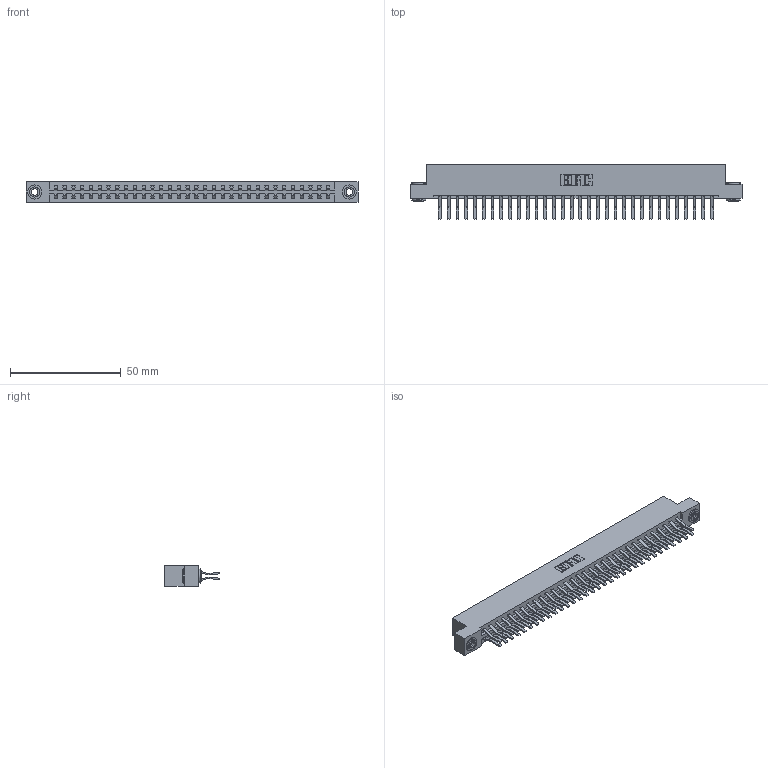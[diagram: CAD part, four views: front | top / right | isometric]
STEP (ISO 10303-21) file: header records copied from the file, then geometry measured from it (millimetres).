
FILE_DESCRIPTION (( 'STEP AP203' ), '1' );
FILE_NAME ('387-064-560-203.STEP', '2019-10-19T17:47:14', ( '' ), ( '' ), 'SwSTEP 2.0', 'SolidWorks 2016', '' );
FILE_SCHEMA (( 'CONFIG_CONTROL_DESIGN' ));
Length unit declared in the file: inch
Products named in the file (4): 345-250-002_345-250-002-102; 387-064-560-203; 337 Part_Flush Mounting Lugs - 0.156 Dia-TH; 345-292-001_560 Tail
Assembly tree (67 placements, depth 2):
  387-064-560-203
    337 Part_Flush Mounting Lugs - 0.156 Dia-TH
    345-292-001_560 Tail  x64
    345-250-002_345-250-002-102  x2
Bounding box: 149.81 x 24.78 x 9.4 mm (x, y, z)
Volume: 16093.9 mm3; surface area: 19535.5 mm2
Topology: 67 solids, 67 shells, 3736 faces, 11075 edges, 7294 vertices
Faces by surface type: plane 2512, cylinder 1216, cone 8
Entity records: 26842 total; most frequent: CARTESIAN_POINT 4505, ORIENTED_EDGE 4434, DIRECTION 3887, EDGE_CURVE 2217, VECTOR 2061, LINE 2061, VERTEX_POINT 1474, AXIS2_PLACEMENT_3D 913
